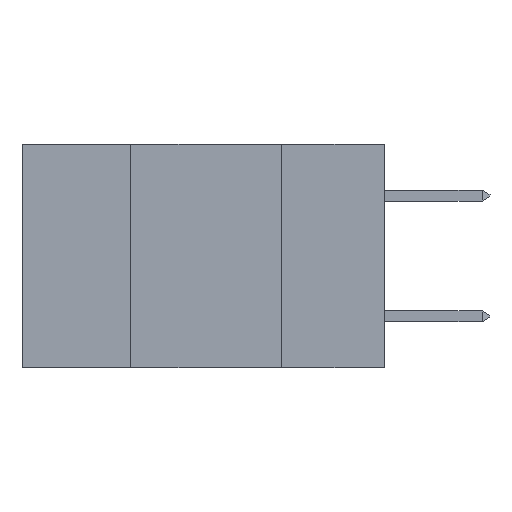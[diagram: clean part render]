
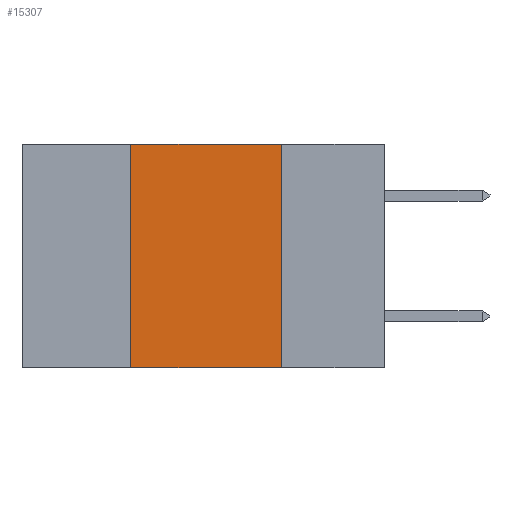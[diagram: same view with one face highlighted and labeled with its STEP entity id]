
A CAD part, left-side view. The second image highlights one B-rep face of the part: STEP entity #15307.
In plain terms, the highlighted planar face has unit normal (-1, 0, 0).
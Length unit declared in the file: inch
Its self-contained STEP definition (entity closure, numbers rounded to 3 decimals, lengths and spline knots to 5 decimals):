
#545 = LINE ( 'NONE', #6992, #14258 ) ;
#3840 = VECTOR ( 'NONE', #10247, 39.37008 ) ;
#5129 = EDGE_CURVE ( 'NONE', #15685, #16048, #19885, .T. ) ;
#5171 = DIRECTION ( 'NONE',  ( 0., 0., -1. ) ) ;
#5403 = ORIENTED_EDGE ( 'NONE', *, *, #11044, .F. ) ;
#6048 = ORIENTED_EDGE ( 'NONE', *, *, #22837, .F. ) ;
#6284 = CARTESIAN_POINT ( 'NONE',  ( 0., 0.6, 0. ) ) ;
#6287 = CARTESIAN_POINT ( 'NONE',  ( 0., 0.6, -0.37 ) ) ;
#6992 = CARTESIAN_POINT ( 'NONE',  ( 0., 0.17, 0. ) ) ;
#7725 = DIRECTION ( 'NONE',  ( 1., 0., 0. ) ) ;
#7886 = VECTOR ( 'NONE', #19688, 39.37008 ) ;
#8137 = ORIENTED_EDGE ( 'NONE', *, *, #5129, .T. ) ;
#8208 = CARTESIAN_POINT ( 'NONE',  ( 0., 0.17, -0.37 ) ) ;
#8781 = LINE ( 'NONE', #19440, #7886 ) ;
#8919 = VERTEX_POINT ( 'NONE', #19023 ) ;
#9119 = AXIS2_PLACEMENT_3D ( 'NONE', #6284, #7725, #13404 ) ;
#9301 = VECTOR ( 'NONE', #23136, 39.37008 ) ;
#10247 = DIRECTION ( 'NONE',  ( 0., -1., 0. ) ) ;
#11044 = EDGE_CURVE ( 'NONE', #15685, #8919, #8781, .T. ) ;
#12271 = EDGE_CURVE ( 'NONE', #8919, #20856, #14248, .T. ) ;
#12635 = FACE_OUTER_BOUND ( 'NONE', #19272, .T. ) ;
#13009 = PLANE ( 'NONE',  #9119 ) ;
#13404 = DIRECTION ( 'NONE',  ( 0., 0., -1. ) ) ;
#14248 = LINE ( 'NONE', #21288, #9301 ) ;
#14258 = VECTOR ( 'NONE', #5171, 39.37008 ) ;
#15307 = ADVANCED_FACE ( 'NONE', ( #12635 ), #13009, .F. ) ;
#15685 = VERTEX_POINT ( 'NONE', #22770 ) ;
#16048 = VERTEX_POINT ( 'NONE', #8208 ) ;
#19023 = CARTESIAN_POINT ( 'NONE',  ( 0., 0.42, 0. ) ) ;
#19272 = EDGE_LOOP ( 'NONE', ( #6048, #20334, #5403, #8137 ) ) ;
#19440 = CARTESIAN_POINT ( 'NONE',  ( 0., 0.42, 0. ) ) ;
#19688 = DIRECTION ( 'NONE',  ( 0., 0., 1. ) ) ;
#19885 = LINE ( 'NONE', #6287, #3840 ) ;
#20334 = ORIENTED_EDGE ( 'NONE', *, *, #12271, .F. ) ;
#20856 = VERTEX_POINT ( 'NONE', #22612 ) ;
#21288 = CARTESIAN_POINT ( 'NONE',  ( 0., 0.6, 0. ) ) ;
#22612 = CARTESIAN_POINT ( 'NONE',  ( 0., 0.17, 0. ) ) ;
#22770 = CARTESIAN_POINT ( 'NONE',  ( 0., 0.42, -0.37 ) ) ;
#22837 = EDGE_CURVE ( 'NONE', #20856, #16048, #545, .T. ) ;
#23136 = DIRECTION ( 'NONE',  ( 0., -1., 0. ) ) ;
